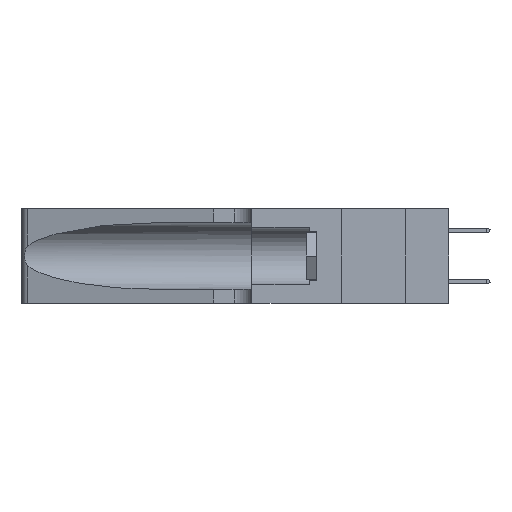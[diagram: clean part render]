
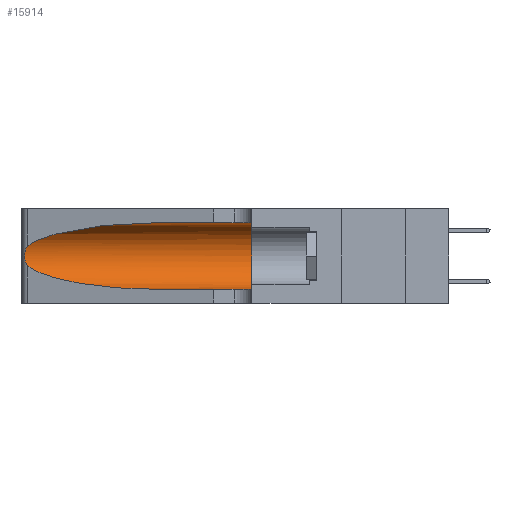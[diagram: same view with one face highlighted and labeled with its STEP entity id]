
A CAD part, left-side view. The second image highlights one B-rep face of the part: STEP entity #15914.
In plain terms, the highlighted cylindrical face has radius 3.308 mm (diameter 6.617 mm), a partial arc.
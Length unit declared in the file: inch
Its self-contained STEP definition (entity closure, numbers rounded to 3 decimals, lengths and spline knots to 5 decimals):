
#1189 = CARTESIAN_POINT ( 'NONE',  ( 0.1305, 1.61858, 0.05475 ) ) ;
#1356 = CARTESIAN_POINT ( 'NONE',  ( 0.25639, 1.23186, 0.15144 ) ) ;
#2491 = CARTESIAN_POINT ( 'NONE',  ( 0.1305, 1.61858, 0.31525 ) ) ;
#3449 = EDGE_CURVE ( 'NONE', #8679, #19883, #30802, .T. ) ;
#3950 = EDGE_CURVE ( 'NONE', #10500, #34131, #9095, .T. ) ;
#4112 = CARTESIAN_POINT ( 'NONE',  ( 0.25555, 1.22994, 0.2215 ) ) ;
#5009 = DIRECTION ( 'NONE',  ( 0., -1., 0. ) ) ;
#6782 = CARTESIAN_POINT ( 'NONE',  ( 0.18966, 0.96281, 0.31525 ) ) ;
#6901 = CARTESIAN_POINT ( 'NONE',  ( 0.25487, 1.22718, 0.14631 ) ) ;
#8607 = ORIENTED_EDGE ( 'NONE', *, *, #30405, .F. ) ;
#8679 = VERTEX_POINT ( 'NONE', #19456 ) ;
#8848 = CARTESIAN_POINT ( 'NONE',  ( 0.1305, 0.35, 0.185 ) ) ;
#9095 = LINE ( 'NONE', #2491, #21730 ) ;
#9709 = CARTESIAN_POINT ( 'NONE',  ( 0.25787, 1.23484, 0.2124 ) ) ;
#10085 = CARTESIAN_POINT ( 'NONE',  ( 0.25639, 1.23184, 0.21858 ) ) ;
#10500 = VERTEX_POINT ( 'NONE', #35108 ) ;
#11395 = ORIENTED_EDGE ( 'NONE', *, *, #33547, .T. ) ;
#12146 = CARTESIAN_POINT ( 'NONE',  ( 0.1305, 1.61858, 0.185 ) ) ;
#12567 = CARTESIAN_POINT ( 'NONE',  ( 0.2373, 1.15595, 0.08982 ) ) ;
#12628 = VERTEX_POINT ( 'NONE', #33706 ) ;
#13166 = CARTESIAN_POINT ( 'NONE',  ( 0.1305, 0.35, 0.31525 ) ) ;
#14259 = DIRECTION ( 'NONE',  ( 0., 1., 0. ) ) ;
#14479 = CARTESIAN_POINT ( 'NONE',  ( 0.25487, 1.22718, 0.22369 ) ) ;
#15085 = ORIENTED_EDGE ( 'NONE', *, *, #20786, .T. ) ;
#15473 = CARTESIAN_POINT ( 'NONE',  ( 0.26018, 1.23835, 0.19895 ) ) ;
#15659 = ORIENTED_EDGE ( 'NONE', *, *, #3449, .T. ) ;
#15824 = CARTESIAN_POINT ( 'NONE',  ( 0.18966, 0.96281, 0.05475 ) ) ;
#15914 = ADVANCED_FACE ( 'NONE', ( #26164 ), #22579, .F. ) ;
#18123 = CARTESIAN_POINT ( 'NONE',  ( 0.1305, 0.72297, 0.31525 ) ) ;
#18362 = ORIENTED_EDGE ( 'NONE', *, *, #3950, .F. ) ;
#18382 = CARTESIAN_POINT ( 'NONE',  ( 0.25789, 1.23486, 0.15765 ) ) ;
#18773 = VECTOR ( 'NONE', #23351, 39.37008 ) ;
#19456 = CARTESIAN_POINT ( 'NONE',  ( 0.25487, 1.22718, 0.14631 ) ) ;
#19883 = VERTEX_POINT ( 'NONE', #25322 ) ;
#20786 = EDGE_CURVE ( 'NONE', #19883, #12628, #34009, .T. ) ;
#21020 = CARTESIAN_POINT ( 'NONE',  ( 0.25487, 1.22718, 0.22369 ) ) ;
#21635 = EDGE_CURVE ( 'NONE', #31331, #8679, #34254, .T. ) ;
#21730 = VECTOR ( 'NONE', #5009, 39.37008 ) ;
#22139 = EDGE_LOOP ( 'NONE', ( #11395, #35153, #15659, #15085, #8607, #18362 ) ) ;
#22579 = CYLINDRICAL_SURFACE ( 'NONE', #36655, 0.13025 ) ;
#23351 = DIRECTION ( 'NONE',  ( 0., -1., 0. ) ) ;
#24061 = CIRCLE ( 'NONE', #30643, 0.13025 ) ;
#24722 = DIRECTION ( 'NONE',  ( 0., 0., -1. ) ) ;
#24977 = DIRECTION ( 'NONE',  ( 0., -1., 0. ) ) ;
#25322 = CARTESIAN_POINT ( 'NONE',  ( 0.1305, 0.72297, 0.05475 ) ) ;
#26164 = FACE_OUTER_BOUND ( 'NONE', #22139, .T. ) ;
#29405 = CARTESIAN_POINT ( 'NONE',  ( 0.2373, 1.15595, 0.28018 ) ) ;
#29646 = CARTESIAN_POINT ( 'NONE',  ( 0.25555, 1.22993, 0.14849 ) ) ;
#29755 = CARTESIAN_POINT ( 'NONE',  ( 0.25487, 1.22718, 0.14631 ) ) ;
#29777 = CARTESIAN_POINT ( 'NONE',  ( 0.26017, 1.23833, 0.17102 ) ) ;
#29905 = CARTESIAN_POINT ( 'NONE',  ( 0.26075, 1.23896, 0.178 ) ) ;
#30145 = CARTESIAN_POINT ( 'NONE',  ( 0.26075, 1.23896, 0.19203 ) ) ;
#30405 = EDGE_CURVE ( 'NONE', #34131, #12628, #24061, .T. ) ;
#30643 = AXIS2_PLACEMENT_3D ( 'NONE', #8848, #14259, #34348 ) ;
#30802 =( BOUNDED_CURVE ( )  B_SPLINE_CURVE ( 3, ( #29755, #12567, #15824, #35943 ),
 .UNSPECIFIED., .F., .F. ) 
 B_SPLINE_CURVE_WITH_KNOTS ( ( 4, 4 ),
 ( 3.44316, 4.71239 ),
 .UNSPECIFIED. ) 
 CURVE ( )  GEOMETRIC_REPRESENTATION_ITEM ( )  RATIONAL_B_SPLINE_CURVE ( ( 1., 0.87, 0.87, 1. ) ) 
 REPRESENTATION_ITEM ( '' )  );
#31331 = VERTEX_POINT ( 'NONE', #14479 ) ;
#31941 =( BOUNDED_CURVE ( )  B_SPLINE_CURVE ( 3, ( #18123, #6782, #29405, #21020 ),
 .UNSPECIFIED., .F., .F. ) 
 B_SPLINE_CURVE_WITH_KNOTS ( ( 4, 4 ),
 ( 1.5708, 2.84003 ),
 .UNSPECIFIED. ) 
 CURVE ( )  GEOMETRIC_REPRESENTATION_ITEM ( )  RATIONAL_B_SPLINE_CURVE ( ( 1., 0.87, 0.87, 1. ) ) 
 REPRESENTATION_ITEM ( '' )  );
#32674 = CARTESIAN_POINT ( 'NONE',  ( 0.25856, 1.23593, 0.16098 ) ) ;
#33547 = EDGE_CURVE ( 'NONE', #10500, #31331, #31941, .T. ) ;
#33706 = CARTESIAN_POINT ( 'NONE',  ( 0.1305, 0.35, 0.05475 ) ) ;
#34009 = LINE ( 'NONE', #1189, #18773 ) ;
#34131 = VERTEX_POINT ( 'NONE', #13166 ) ;
#34254 = B_SPLINE_CURVE_WITH_KNOTS ( 'NONE', 3,
 ( #35704, #4112, #10085, #9709, #35837, #15473, #30145, #29905, #29777, #32674, #18382, #1356, #29646, #6901 ),
 .UNSPECIFIED., .F., .F.,
 ( 4, 2, 2, 2, 2, 2, 4 ),
 ( 0., 0.00027, 0.00053, 0.00107, 0.0016, 0.00187, 0.00214 ),
 .UNSPECIFIED. ) ;
#34348 = DIRECTION ( 'NONE',  ( 0., 0., 1. ) ) ;
#35108 = CARTESIAN_POINT ( 'NONE',  ( 0.1305, 0.72297, 0.31525 ) ) ;
#35153 = ORIENTED_EDGE ( 'NONE', *, *, #21635, .T. ) ;
#35704 = CARTESIAN_POINT ( 'NONE',  ( 0.25487, 1.22718, 0.22369 ) ) ;
#35837 = CARTESIAN_POINT ( 'NONE',  ( 0.25854, 1.2359, 0.20912 ) ) ;
#35943 = CARTESIAN_POINT ( 'NONE',  ( 0.1305, 0.72297, 0.05475 ) ) ;
#36655 = AXIS2_PLACEMENT_3D ( 'NONE', #12146, #24977, #24722 ) ;
